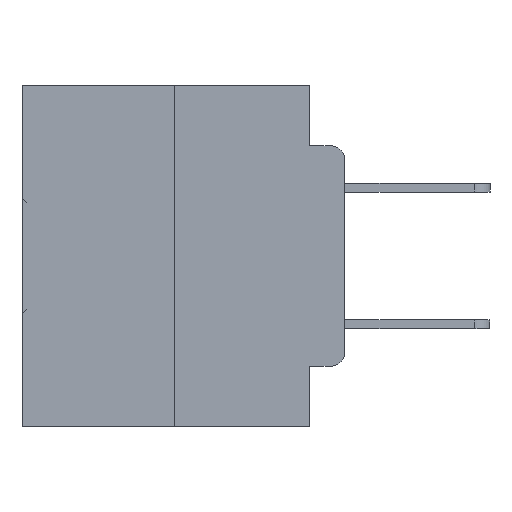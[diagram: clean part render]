
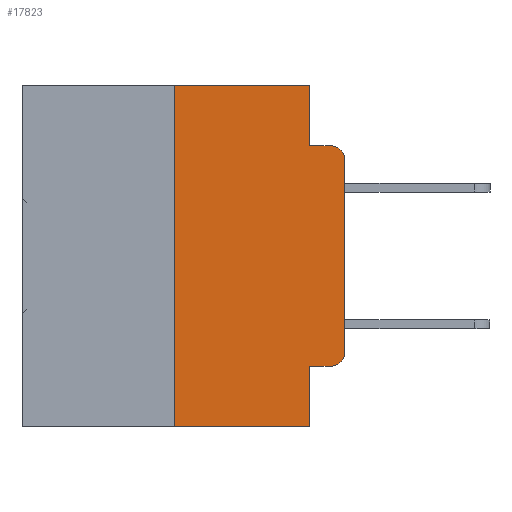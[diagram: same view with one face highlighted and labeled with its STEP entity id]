
A CAD part, left-side view. The second image highlights one B-rep face of the part: STEP entity #17823.
In plain terms, the highlighted planar face has unit normal (-1, 0, 0).
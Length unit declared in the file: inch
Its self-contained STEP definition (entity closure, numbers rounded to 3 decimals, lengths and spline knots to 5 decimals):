
#227 = EDGE_CURVE ( 'NONE', #530, #4506, #31684, .T. ) ;
#251 = LINE ( 'NONE', #16200, #7171 ) ;
#272 = ORIENTED_EDGE ( 'NONE', *, *, #19312, .T. ) ;
#530 = VERTEX_POINT ( 'NONE', #25186 ) ;
#1015 = DIRECTION ( 'NONE',  ( 0., 0., -1. ) ) ;
#1143 = CARTESIAN_POINT ( 'NONE',  ( 0., 0., -0.1085 ) ) ;
#1616 = CARTESIAN_POINT ( 'NONE',  ( 0., 0.473, 0. ) ) ;
#1809 = VERTEX_POINT ( 'NONE', #26791 ) ;
#2073 = VECTOR ( 'NONE', #2709, 39.37008 ) ;
#2224 = DIRECTION ( 'NONE',  ( 0., -1., 0. ) ) ;
#2709 = DIRECTION ( 'NONE',  ( 0., -1., 0. ) ) ;
#2958 = CARTESIAN_POINT ( 'NONE',  ( 0., 0., -0.3915 ) ) ;
#4237 = LINE ( 'NONE', #28714, #23837 ) ;
#4349 = ORIENTED_EDGE ( 'NONE', *, *, #16121, .F. ) ;
#4506 = VERTEX_POINT ( 'NONE', #22886 ) ;
#4611 = VECTOR ( 'NONE', #2224, 39.37008 ) ;
#5201 = EDGE_CURVE ( 'NONE', #15083, #14785, #15849, .T. ) ;
#5717 = LINE ( 'NONE', #24714, #11810 ) ;
#6359 = FACE_OUTER_BOUND ( 'NONE', #18934, .T. ) ;
#6439 = VECTOR ( 'NONE', #25703, 39.37008 ) ;
#7171 = VECTOR ( 'NONE', #28805, 39.37008 ) ;
#7547 = ORIENTED_EDGE ( 'NONE', *, *, #227, .F. ) ;
#7977 = DIRECTION ( 'NONE',  ( 0., 0., -1. ) ) ;
#8281 = ORIENTED_EDGE ( 'NONE', *, *, #28418, .T. ) ;
#8994 = VECTOR ( 'NONE', #7977, 39.37008 ) ;
#9356 = CIRCLE ( 'NONE', #26253, 0.02 ) ;
#9515 = CARTESIAN_POINT ( 'NONE',  ( 0., 0.051, -0.4115 ) ) ;
#9736 = LINE ( 'NONE', #19072, #22464 ) ;
#10480 = CARTESIAN_POINT ( 'NONE',  ( 0., 0.25, 0. ) ) ;
#10750 = EDGE_CURVE ( 'NONE', #27103, #21558, #251, .T. ) ;
#10898 = CARTESIAN_POINT ( 'NONE',  ( 0., 0.02, -0.4115 ) ) ;
#11810 = VECTOR ( 'NONE', #19662, 39.37008 ) ;
#12050 = DIRECTION ( 'NONE',  ( 0., 0., -1. ) ) ;
#12605 = CARTESIAN_POINT ( 'NONE',  ( 0., 0.051, -0.0885 ) ) ;
#12852 = VERTEX_POINT ( 'NONE', #28894 ) ;
#13159 = DIRECTION ( 'NONE',  ( -1., 0., 0. ) ) ;
#13289 = LINE ( 'NONE', #10480, #6439 ) ;
#13350 = AXIS2_PLACEMENT_3D ( 'NONE', #28381, #13159, #30879 ) ;
#13516 = CARTESIAN_POINT ( 'NONE',  ( 0., 0.02, -0.1085 ) ) ;
#14573 = CARTESIAN_POINT ( 'NONE',  ( 0., 0.051, -0.4115 ) ) ;
#14700 = EDGE_CURVE ( 'NONE', #1809, #530, #14997, .T. ) ;
#14785 = VERTEX_POINT ( 'NONE', #10898 ) ;
#14997 = LINE ( 'NONE', #20819, #8994 ) ;
#15083 = VERTEX_POINT ( 'NONE', #14573 ) ;
#15394 = EDGE_CURVE ( 'NONE', #22546, #4506, #9356, .T. ) ;
#15849 = LINE ( 'NONE', #9515, #2073 ) ;
#16121 = EDGE_CURVE ( 'NONE', #27103, #12852, #13289, .T. ) ;
#16131 = DIRECTION ( 'NONE',  ( 0., 0., -1. ) ) ;
#16200 = CARTESIAN_POINT ( 'NONE',  ( 0., 0.473, -0.5 ) ) ;
#16367 = EDGE_CURVE ( 'NONE', #15083, #21558, #9736, .T. ) ;
#17807 = AXIS2_PLACEMENT_3D ( 'NONE', #1616, #27289, #12050 ) ;
#17823 = ADVANCED_FACE ( 'NONE', ( #6359 ), #24705, .F. ) ;
#18934 = EDGE_LOOP ( 'NONE', ( #8281, #23626, #7547, #26908, #25834, #4349, #28379, #32494, #24600, #272 ) ) ;
#19072 = CARTESIAN_POINT ( 'NONE',  ( 0., 0.051, 0. ) ) ;
#19312 = EDGE_CURVE ( 'NONE', #14785, #30823, #21098, .T. ) ;
#19662 = DIRECTION ( 'NONE',  ( 0., 0., 1. ) ) ;
#20819 = CARTESIAN_POINT ( 'NONE',  ( 0., 0.051, 0. ) ) ;
#21098 = CIRCLE ( 'NONE', #13350, 0.02 ) ;
#21558 = VERTEX_POINT ( 'NONE', #32437 ) ;
#22464 = VECTOR ( 'NONE', #1015, 39.37008 ) ;
#22546 = VERTEX_POINT ( 'NONE', #1143 ) ;
#22886 = CARTESIAN_POINT ( 'NONE',  ( 0., 0.02, -0.0885 ) ) ;
#23626 = ORIENTED_EDGE ( 'NONE', *, *, #15394, .T. ) ;
#23837 = VECTOR ( 'NONE', #28835, 39.37008 ) ;
#24600 = ORIENTED_EDGE ( 'NONE', *, *, #5201, .T. ) ;
#24705 = PLANE ( 'NONE',  #17807 ) ;
#24714 = CARTESIAN_POINT ( 'NONE',  ( 0., 0., 0. ) ) ;
#25138 = CARTESIAN_POINT ( 'NONE',  ( 0., 0.25, -0.5 ) ) ;
#25186 = CARTESIAN_POINT ( 'NONE',  ( 0., 0.051, -0.0885 ) ) ;
#25703 = DIRECTION ( 'NONE',  ( 0., 0., 1. ) ) ;
#25834 = ORIENTED_EDGE ( 'NONE', *, *, #26736, .F. ) ;
#26253 = AXIS2_PLACEMENT_3D ( 'NONE', #13516, #31225, #16131 ) ;
#26736 = EDGE_CURVE ( 'NONE', #12852, #1809, #4237, .T. ) ;
#26791 = CARTESIAN_POINT ( 'NONE',  ( 0., 0.051, 0. ) ) ;
#26908 = ORIENTED_EDGE ( 'NONE', *, *, #14700, .F. ) ;
#27103 = VERTEX_POINT ( 'NONE', #25138 ) ;
#27289 = DIRECTION ( 'NONE',  ( 1., 0., 0. ) ) ;
#28379 = ORIENTED_EDGE ( 'NONE', *, *, #10750, .T. ) ;
#28381 = CARTESIAN_POINT ( 'NONE',  ( 0., 0.02, -0.3915 ) ) ;
#28418 = EDGE_CURVE ( 'NONE', #30823, #22546, #5717, .T. ) ;
#28714 = CARTESIAN_POINT ( 'NONE',  ( 0., 0.473, 0. ) ) ;
#28805 = DIRECTION ( 'NONE',  ( 0., -1., 0. ) ) ;
#28835 = DIRECTION ( 'NONE',  ( 0., -1., 0. ) ) ;
#28894 = CARTESIAN_POINT ( 'NONE',  ( 0., 0.25, 0. ) ) ;
#30823 = VERTEX_POINT ( 'NONE', #2958 ) ;
#30879 = DIRECTION ( 'NONE',  ( 0., 0., -1. ) ) ;
#31225 = DIRECTION ( 'NONE',  ( -1., 0., 0. ) ) ;
#31684 = LINE ( 'NONE', #12605, #4611 ) ;
#32437 = CARTESIAN_POINT ( 'NONE',  ( 0., 0.051, -0.5 ) ) ;
#32494 = ORIENTED_EDGE ( 'NONE', *, *, #16367, .F. ) ;
